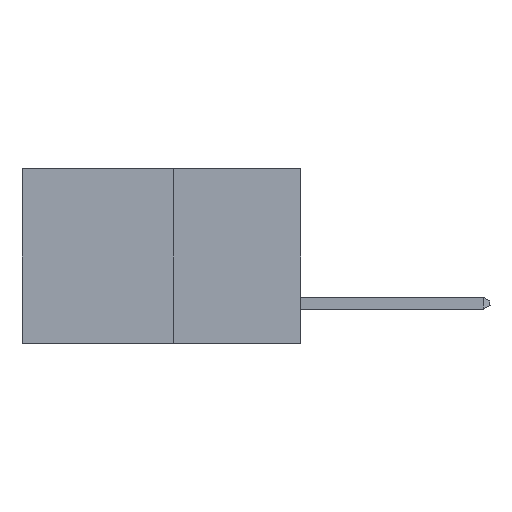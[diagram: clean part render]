
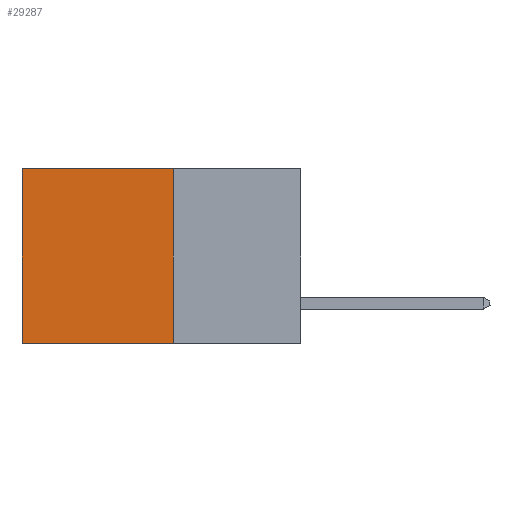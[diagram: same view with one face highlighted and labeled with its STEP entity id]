
A CAD part, left-side view. The second image highlights one B-rep face of the part: STEP entity #29287.
In plain terms, the highlighted planar face has unit normal (-1, 0, 0).
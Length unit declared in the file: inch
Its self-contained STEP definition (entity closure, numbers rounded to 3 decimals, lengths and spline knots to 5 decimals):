
#1229 = VERTEX_POINT ( 'NONE', #27950 ) ;
#1326 = AXIS2_PLACEMENT_3D ( 'NONE', #12846, #29161, #15229 ) ;
#1340 = CARTESIAN_POINT ( 'NONE',  ( 0.277, 0.27, -0.37 ) ) ;
#1392 = VECTOR ( 'NONE', #9829, 39.37008 ) ;
#3181 = DIRECTION ( 'NONE',  ( 0., 1., 0. ) ) ;
#3259 = CARTESIAN_POINT ( 'NONE',  ( 0.277, 0.27, 0. ) ) ;
#3552 = VECTOR ( 'NONE', #25617, 39.37008 ) ;
#3909 = CARTESIAN_POINT ( 'NONE',  ( 0.277, 0.27, -0.37 ) ) ;
#5062 = CARTESIAN_POINT ( 'NONE',  ( 0.277, 0.27, -0.37 ) ) ;
#6754 = VERTEX_POINT ( 'NONE', #3909 ) ;
#6805 = EDGE_CURVE ( 'NONE', #21456, #1229, #13690, .T. ) ;
#6845 = LINE ( 'NONE', #1340, #19386 ) ;
#8766 = EDGE_LOOP ( 'NONE', ( #13211, #14701, #16169, #10631 ) ) ;
#8875 = VERTEX_POINT ( 'NONE', #15915 ) ;
#9193 = CARTESIAN_POINT ( 'NONE',  ( 0.277, 0.59, -0.37 ) ) ;
#9829 = DIRECTION ( 'NONE',  ( 0., 0., -1. ) ) ;
#10631 = ORIENTED_EDGE ( 'NONE', *, *, #6805, .T. ) ;
#10790 = DIRECTION ( 'NONE',  ( 0., 1., 0. ) ) ;
#12846 = CARTESIAN_POINT ( 'NONE',  ( 0.277, 0.27, -0.37 ) ) ;
#13211 = ORIENTED_EDGE ( 'NONE', *, *, #25012, .T. ) ;
#13690 = LINE ( 'NONE', #3259, #19013 ) ;
#14701 = ORIENTED_EDGE ( 'NONE', *, *, #18390, .F. ) ;
#15229 = DIRECTION ( 'NONE',  ( 0., 0., -1. ) ) ;
#15521 = FACE_OUTER_BOUND ( 'NONE', #8766, .T. ) ;
#15915 = CARTESIAN_POINT ( 'NONE',  ( 0.277, 0.59, -0.37 ) ) ;
#16169 = ORIENTED_EDGE ( 'NONE', *, *, #29780, .F. ) ;
#18390 = EDGE_CURVE ( 'NONE', #6754, #8875, #6845, .T. ) ;
#19013 = VECTOR ( 'NONE', #3181, 39.37008 ) ;
#19386 = VECTOR ( 'NONE', #10790, 39.37008 ) ;
#20267 = LINE ( 'NONE', #5062, #1392 ) ;
#20535 = CARTESIAN_POINT ( 'NONE',  ( 0.277, 0.27, 0. ) ) ;
#21456 = VERTEX_POINT ( 'NONE', #20535 ) ;
#22356 = LINE ( 'NONE', #9193, #3552 ) ;
#25012 = EDGE_CURVE ( 'NONE', #1229, #8875, #22356, .T. ) ;
#25617 = DIRECTION ( 'NONE',  ( 0., 0., -1. ) ) ;
#26830 = PLANE ( 'NONE',  #1326 ) ;
#27950 = CARTESIAN_POINT ( 'NONE',  ( 0.277, 0.59, 0. ) ) ;
#29161 = DIRECTION ( 'NONE',  ( 1., 0., 0. ) ) ;
#29287 = ADVANCED_FACE ( 'NONE', ( #15521 ), #26830, .F. ) ;
#29780 = EDGE_CURVE ( 'NONE', #21456, #6754, #20267, .T. ) ;
